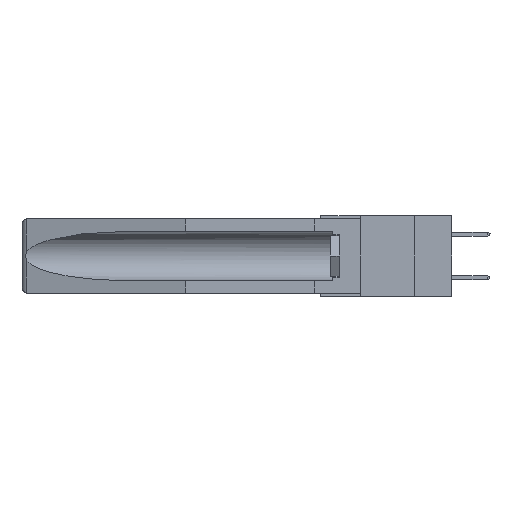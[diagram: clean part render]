
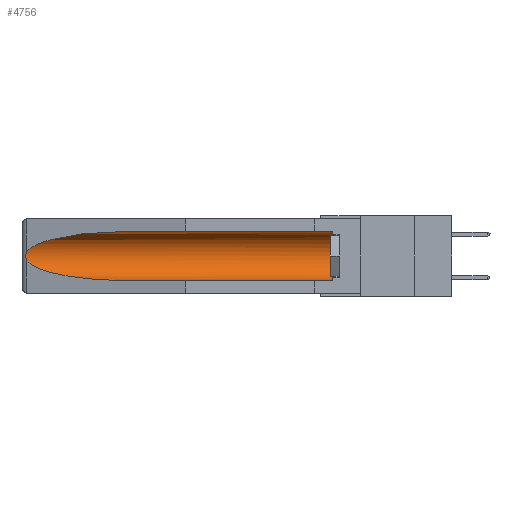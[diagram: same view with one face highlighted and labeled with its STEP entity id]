
A CAD part, left-side view. The second image highlights one B-rep face of the part: STEP entity #4756.
In plain terms, the highlighted cylindrical face has radius 2.857 mm (diameter 5.715 mm), a partial arc.
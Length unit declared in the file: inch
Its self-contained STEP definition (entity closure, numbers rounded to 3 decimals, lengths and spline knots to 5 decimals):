
#48 = DIRECTION ( 'NONE',  ( 0., 1., 0. ) ) ;
#65 = EDGE_CURVE ( 'NONE', #10333, #15488, #7961, .T. ) ;
#233 = CARTESIAN_POINT ( 'NONE',  ( 0.155, 0.126, -0.1715 ) ) ;
#389 = CARTESIAN_POINT ( 'NONE',  ( 0.26655, 1.53094, -0.18657 ) ) ;
#591 = CARTESIAN_POINT ( 'NONE',  ( 0.26597, 1.5296, -0.19026 ) ) ;
#934 = ORIENTED_EDGE ( 'NONE', *, *, #12772, .T. ) ;
#1313 = CARTESIAN_POINT ( 'NONE',  ( 0.155, 1.07973, -0.059 ) ) ;
#1941 = CARTESIAN_POINT ( 'NONE',  ( 0.21114, 1.30732, -0.284 ) ) ;
#2838 = VERTEX_POINT ( 'NONE', #8683 ) ;
#3141 = CARTESIAN_POINT ( 'NONE',  ( 0.155, -0.30754, -0.059 ) ) ;
#3300 = CARTESIAN_POINT ( 'NONE',  ( 0.155, -0.30754, -0.284 ) ) ;
#4477 = DIRECTION ( 'NONE',  ( 0., 1., 0. ) ) ;
#4756 = ADVANCED_FACE ( 'NONE', ( #7728 ), #5091, .F. ) ;
#4900 = CARTESIAN_POINT ( 'NONE',  ( 0.26537, 1.52718, -0.19328 ) ) ;
#5091 = CYLINDRICAL_SURFACE ( 'NONE', #8994, 0.1125 ) ;
#5680 = VERTEX_POINT ( 'NONE', #7928 ) ;
#5743 = ORIENTED_EDGE ( 'NONE', *, *, #9490, .T. ) ;
#6028 = VECTOR ( 'NONE', #48, 39.37008 ) ;
#6294 =( BOUNDED_CURVE ( )  B_SPLINE_CURVE ( 3, ( #4900, #9533, #1941, #14192 ),
 .UNSPECIFIED., .F., .F. ) 
 B_SPLINE_CURVE_WITH_KNOTS ( ( 4, 4 ),
 ( 0.1948, 1.5708 ),
 .UNSPECIFIED. ) 
 CURVE ( )  GEOMETRIC_REPRESENTATION_ITEM ( )  RATIONAL_B_SPLINE_CURVE ( ( 1., 0.848, 0.848, 1. ) ) 
 REPRESENTATION_ITEM ( '' )  );
#6473 = CARTESIAN_POINT ( 'NONE',  ( 0.155, 1.07973, -0.284 ) ) ;
#6570 = AXIS2_PLACEMENT_3D ( 'NONE', #233, #10950, #12386 ) ;
#6817 = EDGE_CURVE ( 'NONE', #10333, #5680, #15046, .T. ) ;
#7728 = FACE_OUTER_BOUND ( 'NONE', #16116, .T. ) ;
#7748 = CARTESIAN_POINT ( 'NONE',  ( 0.26537, 1.52718, -0.19328 ) ) ;
#7840 = DIRECTION ( 'NONE',  ( 0., 1., 0. ) ) ;
#7928 = CARTESIAN_POINT ( 'NONE',  ( 0.155, 0.126, -0.059 ) ) ;
#7961 = LINE ( 'NONE', #3300, #6028 ) ;
#8112 = CARTESIAN_POINT ( 'NONE',  ( 0.26654, 1.53092, -0.15636 ) ) ;
#8175 = CARTESIAN_POINT ( 'NONE',  ( 0.2675, 1.53308, -0.16763 ) ) ;
#8215 = VECTOR ( 'NONE', #7840, 39.37008 ) ;
#8310 = CARTESIAN_POINT ( 'NONE',  ( 0.26537, 1.52718, -0.19328 ) ) ;
#8683 = CARTESIAN_POINT ( 'NONE',  ( 0.26537, 1.52718, -0.14972 ) ) ;
#8923 = DIRECTION ( 'NONE',  ( 0., 0., 1. ) ) ;
#8980 = CARTESIAN_POINT ( 'NONE',  ( 0.21114, 1.30732, -0.059 ) ) ;
#8994 = AXIS2_PLACEMENT_3D ( 'NONE', #16524, #4477, #8923 ) ;
#9490 = EDGE_CURVE ( 'NONE', #13224, #15488, #6294, .T. ) ;
#9533 = CARTESIAN_POINT ( 'NONE',  ( 0.25451, 1.48313, -0.24835 ) ) ;
#10333 = VERTEX_POINT ( 'NONE', #12494 ) ;
#10410 = CARTESIAN_POINT ( 'NONE',  ( 0.25451, 1.48313, -0.09465 ) ) ;
#10482 = ORIENTED_EDGE ( 'NONE', *, *, #6817, .T. ) ;
#10546 = ORIENTED_EDGE ( 'NONE', *, *, #15256, .T. ) ;
#10692 = ORIENTED_EDGE ( 'NONE', *, *, #65, .F. ) ;
#10950 = DIRECTION ( 'NONE',  ( 0., -1., 0. ) ) ;
#11658 = B_SPLINE_CURVE_WITH_KNOTS ( 'NONE', 3,
 ( #18607, #12837, #8112, #17322, #8175, #17256, #17129, #389, #591, #8310 ),
 .UNSPECIFIED., .F., .F.,
 ( 4, 2, 2, 2, 4 ),
 ( 0., 0.00029, 0.00058, 0.00087, 0.00117 ),
 .UNSPECIFIED. ) ;
#12368 = CARTESIAN_POINT ( 'NONE',  ( 0.155, 1.07973, -0.059 ) ) ;
#12386 = DIRECTION ( 'NONE',  ( 0., 0., 1. ) ) ;
#12494 = CARTESIAN_POINT ( 'NONE',  ( 0.155, 0.126, -0.284 ) ) ;
#12772 = EDGE_CURVE ( 'NONE', #14849, #2838, #16240, .T. ) ;
#12837 = CARTESIAN_POINT ( 'NONE',  ( 0.26597, 1.52961, -0.15275 ) ) ;
#13224 = VERTEX_POINT ( 'NONE', #7748 ) ;
#14192 = CARTESIAN_POINT ( 'NONE',  ( 0.155, 1.07973, -0.284 ) ) ;
#14849 = VERTEX_POINT ( 'NONE', #12368 ) ;
#15046 = CIRCLE ( 'NONE', #6570, 0.1125 ) ;
#15256 = EDGE_CURVE ( 'NONE', #2838, #13224, #11658, .T. ) ;
#15488 = VERTEX_POINT ( 'NONE', #6473 ) ;
#15966 = EDGE_CURVE ( 'NONE', #5680, #14849, #17390, .T. ) ;
#16116 = EDGE_LOOP ( 'NONE', ( #934, #10546, #5743, #10692, #10482, #16382 ) ) ;
#16240 =( BOUNDED_CURVE ( )  B_SPLINE_CURVE ( 3, ( #1313, #8980, #10410, #16443 ),
 .UNSPECIFIED., .F., .F. ) 
 B_SPLINE_CURVE_WITH_KNOTS ( ( 4, 4 ),
 ( 4.71239, 6.08839 ),
 .UNSPECIFIED. ) 
 CURVE ( )  GEOMETRIC_REPRESENTATION_ITEM ( )  RATIONAL_B_SPLINE_CURVE ( ( 1., 0.848, 0.848, 1. ) ) 
 REPRESENTATION_ITEM ( '' )  );
#16382 = ORIENTED_EDGE ( 'NONE', *, *, #15966, .T. ) ;
#16443 = CARTESIAN_POINT ( 'NONE',  ( 0.26537, 1.52718, -0.14972 ) ) ;
#16524 = CARTESIAN_POINT ( 'NONE',  ( 0.155, -0.30754, -0.1715 ) ) ;
#17129 = CARTESIAN_POINT ( 'NONE',  ( 0.2673, 1.53269, -0.17917 ) ) ;
#17256 = CARTESIAN_POINT ( 'NONE',  ( 0.2675, 1.53308, -0.17534 ) ) ;
#17322 = CARTESIAN_POINT ( 'NONE',  ( 0.2673, 1.5327, -0.16383 ) ) ;
#17390 = LINE ( 'NONE', #3141, #8215 ) ;
#18607 = CARTESIAN_POINT ( 'NONE',  ( 0.26537, 1.52718, -0.14972 ) ) ;
